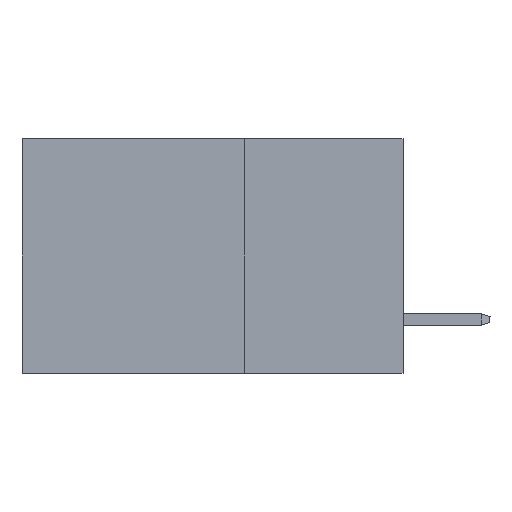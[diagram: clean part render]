
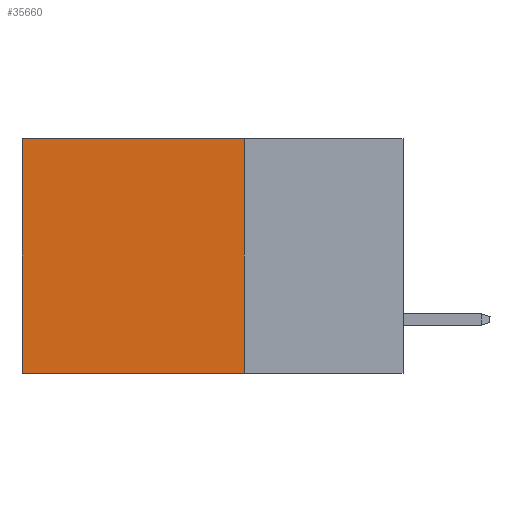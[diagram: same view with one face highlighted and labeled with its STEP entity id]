
A CAD part, left-side view. The second image highlights one B-rep face of the part: STEP entity #35660.
In plain terms, the highlighted planar face has unit normal (-1, 0, 0).
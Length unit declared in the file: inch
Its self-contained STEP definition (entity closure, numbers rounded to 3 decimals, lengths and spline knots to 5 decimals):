
#862 = DIRECTION ( 'NONE',  ( 0., 0., -1. ) ) ;
#1562 = CARTESIAN_POINT ( 'NONE',  ( 0.2875, 0.6, 0. ) ) ;
#2386 = AXIS2_PLACEMENT_3D ( 'NONE', #21251, #21446, #862 ) ;
#4325 = VECTOR ( 'NONE', #34873, 39.37008 ) ;
#4661 = VERTEX_POINT ( 'NONE', #15453 ) ;
#5423 = EDGE_LOOP ( 'NONE', ( #18160, #29727, #20739, #8914 ) ) ;
#5642 = VERTEX_POINT ( 'NONE', #21887 ) ;
#6055 = CARTESIAN_POINT ( 'NONE',  ( 0.2875, 0.6, 0. ) ) ;
#6422 = FACE_OUTER_BOUND ( 'NONE', #5423, .T. ) ;
#8130 = EDGE_CURVE ( 'NONE', #5642, #26278, #36377, .T. ) ;
#8914 = ORIENTED_EDGE ( 'NONE', *, *, #35063, .T. ) ;
#9678 = CARTESIAN_POINT ( 'NONE',  ( 0.2875, 0.25, -0.37 ) ) ;
#10276 = LINE ( 'NONE', #1562, #33865 ) ;
#11617 = VECTOR ( 'NONE', #27074, 39.37008 ) ;
#12249 = EDGE_CURVE ( 'NONE', #14224, #26278, #10276, .T. ) ;
#12540 = PLANE ( 'NONE',  #2386 ) ;
#13505 = LINE ( 'NONE', #25960, #4325 ) ;
#14224 = VERTEX_POINT ( 'NONE', #6055 ) ;
#15453 = CARTESIAN_POINT ( 'NONE',  ( 0.2875, 0.25, 0. ) ) ;
#16946 = DIRECTION ( 'NONE',  ( 0., 1., 0. ) ) ;
#18160 = ORIENTED_EDGE ( 'NONE', *, *, #12249, .T. ) ;
#20739 = ORIENTED_EDGE ( 'NONE', *, *, #35791, .F. ) ;
#21251 = CARTESIAN_POINT ( 'NONE',  ( 0.2875, 0.25, 0. ) ) ;
#21446 = DIRECTION ( 'NONE',  ( 1., 0., 0. ) ) ;
#21887 = CARTESIAN_POINT ( 'NONE',  ( 0.2875, 0.25, -0.37 ) ) ;
#22135 = DIRECTION ( 'NONE',  ( 0., 0., -1. ) ) ;
#25109 = VECTOR ( 'NONE', #16946, 39.37008 ) ;
#25960 = CARTESIAN_POINT ( 'NONE',  ( 0.2875, 0.25, 0. ) ) ;
#26278 = VERTEX_POINT ( 'NONE', #28754 ) ;
#27074 = DIRECTION ( 'NONE',  ( 0., 1., 0. ) ) ;
#28754 = CARTESIAN_POINT ( 'NONE',  ( 0.2875, 0.6, -0.37 ) ) ;
#29727 = ORIENTED_EDGE ( 'NONE', *, *, #8130, .F. ) ;
#33865 = VECTOR ( 'NONE', #22135, 39.37008 ) ;
#34873 = DIRECTION ( 'NONE',  ( 0., 0., -1. ) ) ;
#35063 = EDGE_CURVE ( 'NONE', #4661, #14224, #35163, .T. ) ;
#35163 = LINE ( 'NONE', #38143, #25109 ) ;
#35660 = ADVANCED_FACE ( 'NONE', ( #6422 ), #12540, .F. ) ;
#35791 = EDGE_CURVE ( 'NONE', #4661, #5642, #13505, .T. ) ;
#36377 = LINE ( 'NONE', #9678, #11617 ) ;
#38143 = CARTESIAN_POINT ( 'NONE',  ( 0.2875, 0.25, 0. ) ) ;
